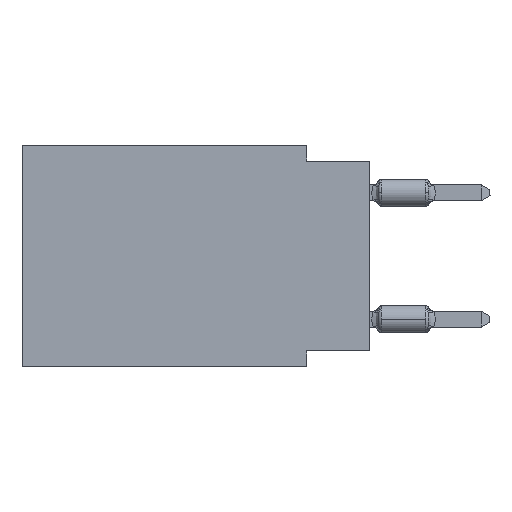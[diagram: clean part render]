
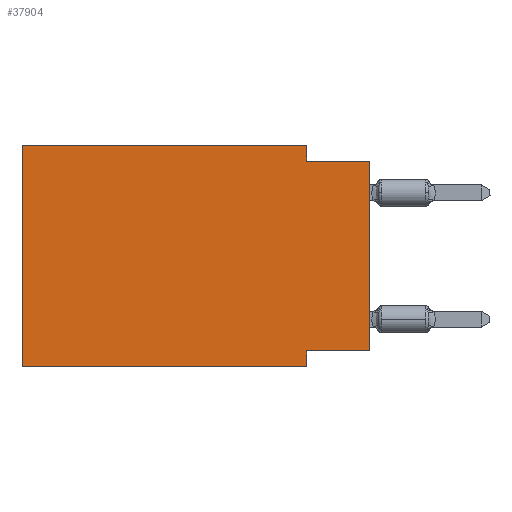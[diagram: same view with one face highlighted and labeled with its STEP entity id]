
A CAD part, left-side view. The second image highlights one B-rep face of the part: STEP entity #37904.
In plain terms, the highlighted planar face has unit normal (-1, 0, 0).
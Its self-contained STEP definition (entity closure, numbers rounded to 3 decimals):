
#1312 = CARTESIAN_POINT ( 'NONE',  ( 0., 2.54, 0. ) ) ;
#2290 = CARTESIAN_POINT ( 'NONE',  ( 0., 0., -8.255 ) ) ;
#4005 = VECTOR ( 'NONE', #24071, 1000. ) ;
#5464 = VECTOR ( 'NONE', #9925, 1000. ) ;
#8103 = LINE ( 'NONE', #16572, #48242 ) ;
#8107 = EDGE_LOOP ( 'NONE', ( #15923, #34009, #32482, #59280, #52738, #26680, #9445, #12298 ) ) ;
#8154 = LINE ( 'NONE', #37072, #4005 ) ;
#9445 = ORIENTED_EDGE ( 'NONE', *, *, #55302, .F. ) ;
#9925 = DIRECTION ( 'NONE',  ( 0., 0., 1. ) ) ;
#10878 = CARTESIAN_POINT ( 'NONE',  ( 0., 2.54, -0.635 ) ) ;
#11274 = EDGE_CURVE ( 'NONE', #47242, #57087, #8154, .T. ) ;
#12298 = ORIENTED_EDGE ( 'NONE', *, *, #11274, .F. ) ;
#13718 = CARTESIAN_POINT ( 'NONE',  ( 0., 2.54, -8.89 ) ) ;
#14262 = CARTESIAN_POINT ( 'NONE',  ( 0., 13.97, 0. ) ) ;
#14705 = VERTEX_POINT ( 'NONE', #30524 ) ;
#15218 = DIRECTION ( 'NONE',  ( 0., 0., -1. ) ) ;
#15576 = CARTESIAN_POINT ( 'NONE',  ( 0., 13.97, -8.89 ) ) ;
#15923 = ORIENTED_EDGE ( 'NONE', *, *, #41676, .T. ) ;
#16277 = CARTESIAN_POINT ( 'NONE',  ( 0., 2.54, -8.255 ) ) ;
#16572 = CARTESIAN_POINT ( 'NONE',  ( 0., 2.54, 0. ) ) ;
#17610 = DIRECTION ( 'NONE',  ( 0., 0., 1. ) ) ;
#18497 = LINE ( 'NONE', #32410, #49719 ) ;
#19160 = DIRECTION ( 'NONE',  ( 1., 0., 0. ) ) ;
#19423 = LINE ( 'NONE', #24253, #23661 ) ;
#19760 = PLANE ( 'NONE',  #26849 ) ;
#19822 = DIRECTION ( 'NONE',  ( 0., -1., 0. ) ) ;
#21069 = VECTOR ( 'NONE', #56287, 1000. ) ;
#21714 = DIRECTION ( 'NONE',  ( 0., 0., -1. ) ) ;
#22806 = EDGE_CURVE ( 'NONE', #46950, #36663, #55604, .T. ) ;
#23441 = DIRECTION ( 'NONE',  ( 0., -1., 0. ) ) ;
#23661 = VECTOR ( 'NONE', #46648, 1000. ) ;
#24071 = DIRECTION ( 'NONE',  ( 0., 1., 0. ) ) ;
#24253 = CARTESIAN_POINT ( 'NONE',  ( 0., 13.97, 0. ) ) ;
#24748 = VERTEX_POINT ( 'NONE', #13718 ) ;
#25897 = EDGE_CURVE ( 'NONE', #47738, #30663, #8103, .T. ) ;
#26680 = ORIENTED_EDGE ( 'NONE', *, *, #52414, .T. ) ;
#26849 = AXIS2_PLACEMENT_3D ( 'NONE', #56672, #19160, #15218 ) ;
#29785 = LINE ( 'NONE', #15576, #54730 ) ;
#30524 = CARTESIAN_POINT ( 'NONE',  ( 0., 0., -0.635 ) ) ;
#30663 = VERTEX_POINT ( 'NONE', #10878 ) ;
#31304 = EDGE_CURVE ( 'NONE', #30663, #14705, #31643, .T. ) ;
#31643 = LINE ( 'NONE', #36746, #48522 ) ;
#32410 = CARTESIAN_POINT ( 'NONE',  ( 0., 0., 0. ) ) ;
#32482 = ORIENTED_EDGE ( 'NONE', *, *, #25897, .F. ) ;
#32764 = FACE_OUTER_BOUND ( 'NONE', #8107, .T. ) ;
#33294 = CARTESIAN_POINT ( 'NONE',  ( 0., 2.54, -8.89 ) ) ;
#34009 = ORIENTED_EDGE ( 'NONE', *, *, #31304, .F. ) ;
#36663 = VERTEX_POINT ( 'NONE', #14262 ) ;
#36746 = CARTESIAN_POINT ( 'NONE',  ( 0., 0., -0.635 ) ) ;
#37072 = CARTESIAN_POINT ( 'NONE',  ( 0., 0., -8.255 ) ) ;
#37904 = ADVANCED_FACE ( 'NONE', ( #32764 ), #19760, .F. ) ;
#41676 = EDGE_CURVE ( 'NONE', #47242, #14705, #18497, .T. ) ;
#46648 = DIRECTION ( 'NONE',  ( 0., -1., 0. ) ) ;
#46841 = CARTESIAN_POINT ( 'NONE',  ( 0., 13.97, 0. ) ) ;
#46950 = VERTEX_POINT ( 'NONE', #49262 ) ;
#47242 = VERTEX_POINT ( 'NONE', #2290 ) ;
#47738 = VERTEX_POINT ( 'NONE', #1312 ) ;
#48242 = VECTOR ( 'NONE', #21714, 1000. ) ;
#48522 = VECTOR ( 'NONE', #23441, 1000. ) ;
#49262 = CARTESIAN_POINT ( 'NONE',  ( 0., 13.97, -8.89 ) ) ;
#49719 = VECTOR ( 'NONE', #17610, 1000. ) ;
#52414 = EDGE_CURVE ( 'NONE', #46950, #24748, #29785, .T. ) ;
#52738 = ORIENTED_EDGE ( 'NONE', *, *, #22806, .F. ) ;
#52955 = LINE ( 'NONE', #33294, #21069 ) ;
#54730 = VECTOR ( 'NONE', #19822, 1000. ) ;
#55302 = EDGE_CURVE ( 'NONE', #57087, #24748, #52955, .T. ) ;
#55604 = LINE ( 'NONE', #46841, #5464 ) ;
#56287 = DIRECTION ( 'NONE',  ( 0., 0., -1. ) ) ;
#56672 = CARTESIAN_POINT ( 'NONE',  ( 0., 13.97, 0. ) ) ;
#57087 = VERTEX_POINT ( 'NONE', #16277 ) ;
#58134 = EDGE_CURVE ( 'NONE', #36663, #47738, #19423, .T. ) ;
#59280 = ORIENTED_EDGE ( 'NONE', *, *, #58134, .F. ) ;
